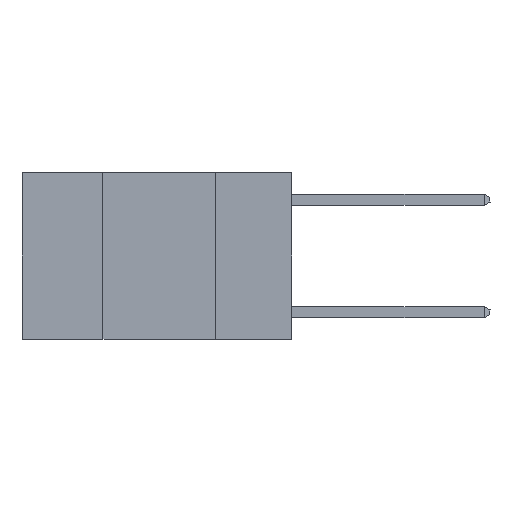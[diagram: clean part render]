
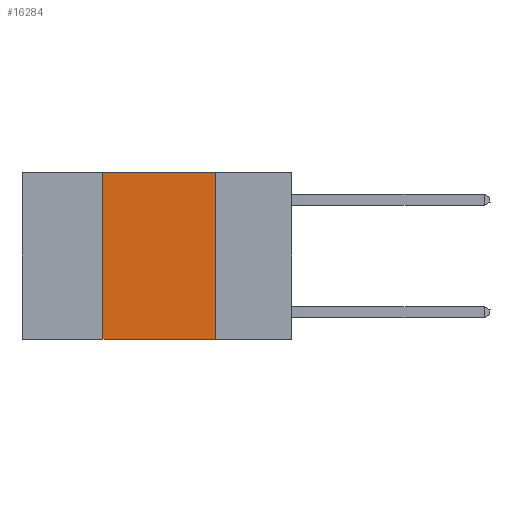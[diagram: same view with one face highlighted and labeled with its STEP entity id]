
A CAD part, left-side view. The second image highlights one B-rep face of the part: STEP entity #16284.
In plain terms, the highlighted planar face has unit normal (-1, 0, 0).
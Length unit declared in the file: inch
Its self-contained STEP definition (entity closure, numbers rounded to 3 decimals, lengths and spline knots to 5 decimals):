
#1276 = EDGE_LOOP ( 'NONE', ( #19791, #21326, #22988, #13352 ) ) ;
#1372 = FACE_OUTER_BOUND ( 'NONE', #1276, .T. ) ;
#3342 = LINE ( 'NONE', #27732, #20465 ) ;
#3677 = CARTESIAN_POINT ( 'NONE',  ( 0., 0.17, 0. ) ) ;
#4414 = DIRECTION ( 'NONE',  ( 0., 0., -1. ) ) ;
#4463 = CARTESIAN_POINT ( 'NONE',  ( 0., 0.6, 0. ) ) ;
#5574 = DIRECTION ( 'NONE',  ( 0., 0., 1. ) ) ;
#5679 = CARTESIAN_POINT ( 'NONE',  ( 0., 0.17, 0. ) ) ;
#8084 = EDGE_CURVE ( 'NONE', #24564, #23874, #3342, .T. ) ;
#8191 = CARTESIAN_POINT ( 'NONE',  ( 0., 0.6, 0. ) ) ;
#9239 = VERTEX_POINT ( 'NONE', #3677 ) ;
#9615 = EDGE_CURVE ( 'NONE', #9239, #23874, #19440, .T. ) ;
#10604 = DIRECTION ( 'NONE',  ( 0., 0., -1. ) ) ;
#11026 = DIRECTION ( 'NONE',  ( 0., -1., 0. ) ) ;
#13352 = ORIENTED_EDGE ( 'NONE', *, *, #8084, .T. ) ;
#14035 = VECTOR ( 'NONE', #10604, 39.37008 ) ;
#15251 = CARTESIAN_POINT ( 'NONE',  ( 0., 0.42, 0. ) ) ;
#16036 = LINE ( 'NONE', #4463, #27291 ) ;
#16162 = EDGE_CURVE ( 'NONE', #24564, #17586, #25326, .T. ) ;
#16284 = ADVANCED_FACE ( 'NONE', ( #1372 ), #19320, .F. ) ;
#17300 = DIRECTION ( 'NONE',  ( 1., 0., 0. ) ) ;
#17586 = VERTEX_POINT ( 'NONE', #15251 ) ;
#17700 = CARTESIAN_POINT ( 'NONE',  ( 0., 0.42, -0.37 ) ) ;
#18073 = DIRECTION ( 'NONE',  ( 0., -1., 0. ) ) ;
#18821 = AXIS2_PLACEMENT_3D ( 'NONE', #8191, #17300, #4414 ) ;
#19320 = PLANE ( 'NONE',  #18821 ) ;
#19440 = LINE ( 'NONE', #5679, #14035 ) ;
#19471 = CARTESIAN_POINT ( 'NONE',  ( 0., 0.17, -0.37 ) ) ;
#19791 = ORIENTED_EDGE ( 'NONE', *, *, #9615, .F. ) ;
#20138 = EDGE_CURVE ( 'NONE', #17586, #9239, #16036, .T. ) ;
#20465 = VECTOR ( 'NONE', #11026, 39.37008 ) ;
#21326 = ORIENTED_EDGE ( 'NONE', *, *, #20138, .F. ) ;
#22988 = ORIENTED_EDGE ( 'NONE', *, *, #16162, .F. ) ;
#23874 = VERTEX_POINT ( 'NONE', #19471 ) ;
#23983 = VECTOR ( 'NONE', #5574, 39.37008 ) ;
#24564 = VERTEX_POINT ( 'NONE', #17700 ) ;
#25182 = CARTESIAN_POINT ( 'NONE',  ( 0., 0.42, 0. ) ) ;
#25326 = LINE ( 'NONE', #25182, #23983 ) ;
#27291 = VECTOR ( 'NONE', #18073, 39.37008 ) ;
#27732 = CARTESIAN_POINT ( 'NONE',  ( 0., 0.6, -0.37 ) ) ;
